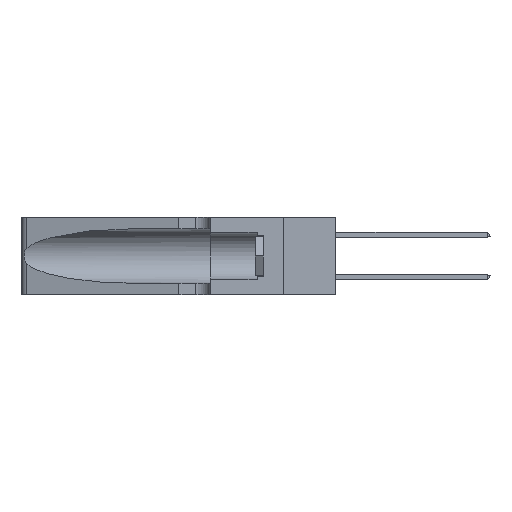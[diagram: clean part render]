
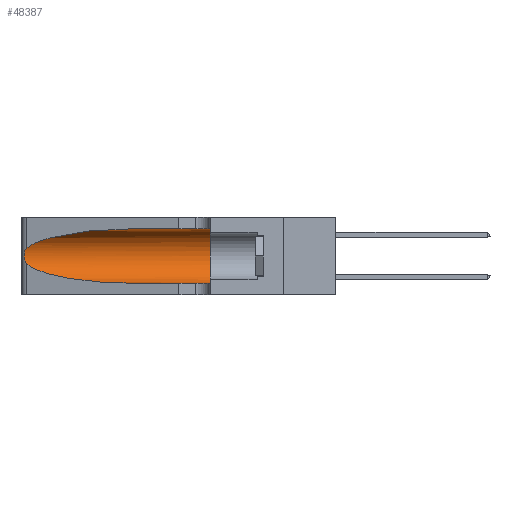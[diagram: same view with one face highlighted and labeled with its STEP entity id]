
A CAD part, left-side view. The second image highlights one B-rep face of the part: STEP entity #48387.
In plain terms, the highlighted cylindrical face has radius 3.308 mm (diameter 6.617 mm), a partial arc.
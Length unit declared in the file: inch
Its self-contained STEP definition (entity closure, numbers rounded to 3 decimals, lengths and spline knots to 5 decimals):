
#1312 = EDGE_CURVE ( 'NONE', #42317, #47262, #10737, .T. ) ;
#2064 = DIRECTION ( 'NONE',  ( 0., -1., 0. ) ) ;
#2216 = ORIENTED_EDGE ( 'NONE', *, *, #35876, .T. ) ;
#2877 = CARTESIAN_POINT ( 'NONE',  ( 0.25487, 1.22718, 0.14631 ) ) ;
#3185 = CARTESIAN_POINT ( 'NONE',  ( 0.25487, 1.22718, 0.22369 ) ) ;
#3433 = CARTESIAN_POINT ( 'NONE',  ( 0.26075, 1.23896, 0.178 ) ) ;
#3769 = LINE ( 'NONE', #7575, #12790 ) ;
#3959 = VECTOR ( 'NONE', #21625, 39.37008 ) ;
#6318 = AXIS2_PLACEMENT_3D ( 'NONE', #32553, #2064, #40024 ) ;
#6376 = ORIENTED_EDGE ( 'NONE', *, *, #43224, .T. ) ;
#6619 = AXIS2_PLACEMENT_3D ( 'NONE', #38701, #15963, #42520 ) ;
#7293 = CARTESIAN_POINT ( 'NONE',  ( 0.25856, 1.23593, 0.16098 ) ) ;
#7575 = CARTESIAN_POINT ( 'NONE',  ( 0.1305, 1.61858, 0.31525 ) ) ;
#8238 = CARTESIAN_POINT ( 'NONE',  ( 0.25487, 1.22718, 0.14631 ) ) ;
#9216 = VERTEX_POINT ( 'NONE', #47337 ) ;
#10737 = B_SPLINE_CURVE_WITH_KNOTS ( 'NONE', 3,
 ( #41381, #11009, #14821, #45180, #22480, #48968, #26272, #3433, #30097, #7293, #33905, #11171, #37729, #14991 ),
 .UNSPECIFIED., .F., .F.,
 ( 4, 2, 2, 2, 2, 2, 4 ),
 ( 0., 0.00027, 0.00053, 0.00107, 0.0016, 0.00187, 0.00214 ),
 .UNSPECIFIED. ) ;
#11009 = CARTESIAN_POINT ( 'NONE',  ( 0.25555, 1.22994, 0.2215 ) ) ;
#11171 = CARTESIAN_POINT ( 'NONE',  ( 0.25639, 1.23186, 0.15144 ) ) ;
#11259 = VERTEX_POINT ( 'NONE', #34931 ) ;
#12274 =( BOUNDED_CURVE ( )  B_SPLINE_CURVE ( 3, ( #2877, #36843, #37173, #14441 ),
 .UNSPECIFIED., .F., .F. ) 
 B_SPLINE_CURVE_WITH_KNOTS ( ( 4, 4 ),
 ( 3.44316, 4.71239 ),
 .UNSPECIFIED. ) 
 CURVE ( )  GEOMETRIC_REPRESENTATION_ITEM ( )  RATIONAL_B_SPLINE_CURVE ( ( 1., 0.87, 0.87, 1. ) ) 
 REPRESENTATION_ITEM ( '' )  );
#12437 = EDGE_LOOP ( 'NONE', ( #2216, #23409, #6376, #39790, #29830, #46098 ) ) ;
#12790 = VECTOR ( 'NONE', #45452, 39.37008 ) ;
#14441 = CARTESIAN_POINT ( 'NONE',  ( 0.1305, 0.72297, 0.05475 ) ) ;
#14585 = CARTESIAN_POINT ( 'NONE',  ( 0.18966, 0.96281, 0.31525 ) ) ;
#14821 = CARTESIAN_POINT ( 'NONE',  ( 0.25639, 1.23184, 0.21858 ) ) ;
#14991 = CARTESIAN_POINT ( 'NONE',  ( 0.25487, 1.22718, 0.14631 ) ) ;
#15356 = LINE ( 'NONE', #17813, #3959 ) ;
#15963 = DIRECTION ( 'NONE',  ( 0., 1., 0. ) ) ;
#17198 = CARTESIAN_POINT ( 'NONE',  ( 0.25487, 1.22718, 0.22369 ) ) ;
#17786 = EDGE_CURVE ( 'NONE', #17946, #11259, #46385, .T. ) ;
#17813 = CARTESIAN_POINT ( 'NONE',  ( 0.1305, 1.61858, 0.05475 ) ) ;
#17946 = VERTEX_POINT ( 'NONE', #24427 ) ;
#21625 = DIRECTION ( 'NONE',  ( 0., -1., 0. ) ) ;
#21757 = CARTESIAN_POINT ( 'NONE',  ( 0.1305, 0.72297, 0.31525 ) ) ;
#22480 = CARTESIAN_POINT ( 'NONE',  ( 0.25854, 1.2359, 0.20912 ) ) ;
#23409 = ORIENTED_EDGE ( 'NONE', *, *, #1312, .T. ) ;
#24427 = CARTESIAN_POINT ( 'NONE',  ( 0.1305, 0.35, 0.31525 ) ) ;
#26030 = CARTESIAN_POINT ( 'NONE',  ( 0.2373, 1.15595, 0.28018 ) ) ;
#26272 = CARTESIAN_POINT ( 'NONE',  ( 0.26075, 1.23896, 0.19203 ) ) ;
#27609 = EDGE_CURVE ( 'NONE', #9216, #11259, #15356, .T. ) ;
#29830 = ORIENTED_EDGE ( 'NONE', *, *, #17786, .F. ) ;
#30097 = CARTESIAN_POINT ( 'NONE',  ( 0.26017, 1.23833, 0.17102 ) ) ;
#32553 = CARTESIAN_POINT ( 'NONE',  ( 0.1305, 1.61858, 0.185 ) ) ;
#33905 = CARTESIAN_POINT ( 'NONE',  ( 0.25789, 1.23486, 0.15765 ) ) ;
#34931 = CARTESIAN_POINT ( 'NONE',  ( 0.1305, 0.35, 0.05475 ) ) ;
#35876 = EDGE_CURVE ( 'NONE', #37681, #42317, #38744, .T. ) ;
#36272 = CYLINDRICAL_SURFACE ( 'NONE', #6318, 0.13025 ) ;
#36843 = CARTESIAN_POINT ( 'NONE',  ( 0.2373, 1.15595, 0.08982 ) ) ;
#37173 = CARTESIAN_POINT ( 'NONE',  ( 0.18966, 0.96281, 0.05475 ) ) ;
#37681 = VERTEX_POINT ( 'NONE', #21757 ) ;
#37729 = CARTESIAN_POINT ( 'NONE',  ( 0.25555, 1.22993, 0.14849 ) ) ;
#38653 = FACE_OUTER_BOUND ( 'NONE', #12437, .T. ) ;
#38701 = CARTESIAN_POINT ( 'NONE',  ( 0.1305, 0.35, 0.185 ) ) ;
#38744 =( BOUNDED_CURVE ( )  B_SPLINE_CURVE ( 3, ( #41141, #14585, #26030, #3185 ),
 .UNSPECIFIED., .F., .F. ) 
 B_SPLINE_CURVE_WITH_KNOTS ( ( 4, 4 ),
 ( 1.5708, 2.84003 ),
 .UNSPECIFIED. ) 
 CURVE ( )  GEOMETRIC_REPRESENTATION_ITEM ( )  RATIONAL_B_SPLINE_CURVE ( ( 1., 0.87, 0.87, 1. ) ) 
 REPRESENTATION_ITEM ( '' )  );
#39790 = ORIENTED_EDGE ( 'NONE', *, *, #27609, .T. ) ;
#40024 = DIRECTION ( 'NONE',  ( 0., 0., -1. ) ) ;
#41141 = CARTESIAN_POINT ( 'NONE',  ( 0.1305, 0.72297, 0.31525 ) ) ;
#41381 = CARTESIAN_POINT ( 'NONE',  ( 0.25487, 1.22718, 0.22369 ) ) ;
#42317 = VERTEX_POINT ( 'NONE', #17198 ) ;
#42520 = DIRECTION ( 'NONE',  ( 0., 0., 1. ) ) ;
#43224 = EDGE_CURVE ( 'NONE', #47262, #9216, #12274, .T. ) ;
#45172 = EDGE_CURVE ( 'NONE', #37681, #17946, #3769, .T. ) ;
#45180 = CARTESIAN_POINT ( 'NONE',  ( 0.25787, 1.23484, 0.2124 ) ) ;
#45452 = DIRECTION ( 'NONE',  ( 0., -1., 0. ) ) ;
#46098 = ORIENTED_EDGE ( 'NONE', *, *, #45172, .F. ) ;
#46385 = CIRCLE ( 'NONE', #6619, 0.13025 ) ;
#47262 = VERTEX_POINT ( 'NONE', #8238 ) ;
#47337 = CARTESIAN_POINT ( 'NONE',  ( 0.1305, 0.72297, 0.05475 ) ) ;
#48387 = ADVANCED_FACE ( 'NONE', ( #38653 ), #36272, .F. ) ;
#48968 = CARTESIAN_POINT ( 'NONE',  ( 0.26018, 1.23835, 0.19895 ) ) ;
